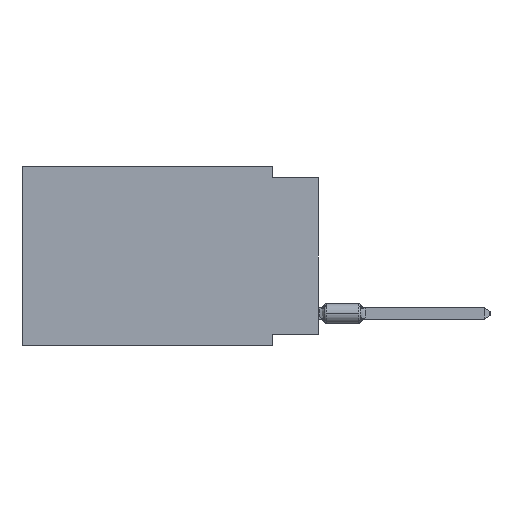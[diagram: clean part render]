
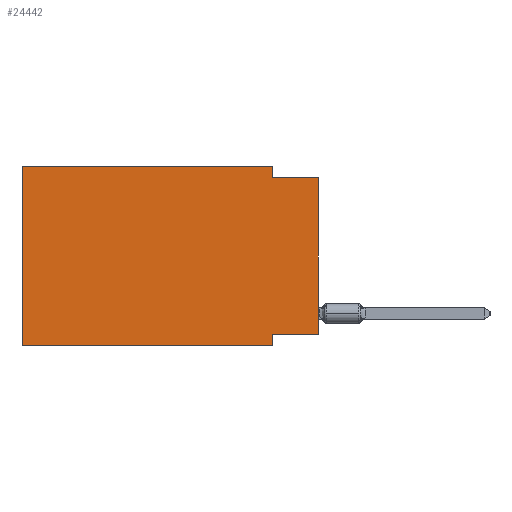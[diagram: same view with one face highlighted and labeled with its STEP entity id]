
A CAD part, left-side view. The second image highlights one B-rep face of the part: STEP entity #24442.
In plain terms, the highlighted planar face has unit normal (-1, 0, 0).
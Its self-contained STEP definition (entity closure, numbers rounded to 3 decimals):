
#1046 = AXIS2_PLACEMENT_3D ( 'NONE', #39281, #25412, #35504 ) ;
#1275 = CARTESIAN_POINT ( 'NONE',  ( 0., 16.383, 0. ) ) ;
#1671 = EDGE_CURVE ( 'NONE', #38551, #7655, #11116, .T. ) ;
#2085 = DIRECTION ( 'NONE',  ( 0., 0., 1. ) ) ;
#3081 = EDGE_CURVE ( 'NONE', #30205, #43479, #19618, .T. ) ;
#3796 = EDGE_CURVE ( 'NONE', #30205, #14501, #11627, .T. ) ;
#4505 = DIRECTION ( 'NONE',  ( 0., -1., 0. ) ) ;
#5519 = CARTESIAN_POINT ( 'NONE',  ( 0., 0., 0. ) ) ;
#6360 = CARTESIAN_POINT ( 'NONE',  ( 0., 2.54, -9.906 ) ) ;
#7655 = VERTEX_POINT ( 'NONE', #32848 ) ;
#8376 = FACE_OUTER_BOUND ( 'NONE', #14781, .T. ) ;
#8791 = CARTESIAN_POINT ( 'NONE',  ( 0., 2.54, 0. ) ) ;
#9458 = LINE ( 'NONE', #32788, #31918 ) ;
#10116 = CARTESIAN_POINT ( 'NONE',  ( 0., 2.54, -0.635 ) ) ;
#11116 = LINE ( 'NONE', #42030, #40801 ) ;
#11627 = LINE ( 'NONE', #22161, #36721 ) ;
#11852 = DIRECTION ( 'NONE',  ( 0., 1., 0. ) ) ;
#12559 = VECTOR ( 'NONE', #4505, 1000. ) ;
#12572 = VERTEX_POINT ( 'NONE', #10116 ) ;
#14501 = VERTEX_POINT ( 'NONE', #23857 ) ;
#14781 = EDGE_LOOP ( 'NONE', ( #31354, #17717, #36612, #36747, #33207, #42353, #42461, #24966 ) ) ;
#16635 = VECTOR ( 'NONE', #26085, 1000. ) ;
#17512 = LINE ( 'NONE', #41033, #32319 ) ;
#17717 = ORIENTED_EDGE ( 'NONE', *, *, #43012, .F. ) ;
#18783 = CARTESIAN_POINT ( 'NONE',  ( 0., 16.383, -9.906 ) ) ;
#19618 = LINE ( 'NONE', #5519, #23778 ) ;
#22090 = DIRECTION ( 'NONE',  ( 0., -1., 0. ) ) ;
#22161 = CARTESIAN_POINT ( 'NONE',  ( 0., 0., -9.271 ) ) ;
#23270 = EDGE_CURVE ( 'NONE', #14501, #30588, #39729, .T. ) ;
#23373 = DIRECTION ( 'NONE',  ( 0., 0., -1. ) ) ;
#23778 = VECTOR ( 'NONE', #25686, 1000. ) ;
#23857 = CARTESIAN_POINT ( 'NONE',  ( 0., 2.54, -9.271 ) ) ;
#23924 = CARTESIAN_POINT ( 'NONE',  ( 0., 0., -0.635 ) ) ;
#24442 = ADVANCED_FACE ( 'NONE', ( #8376 ), #35705, .F. ) ;
#24966 = ORIENTED_EDGE ( 'NONE', *, *, #3796, .F. ) ;
#25412 = DIRECTION ( 'NONE',  ( 1., 0., 0. ) ) ;
#25579 = VECTOR ( 'NONE', #23373, 1000. ) ;
#25686 = DIRECTION ( 'NONE',  ( 0., 0., 1. ) ) ;
#26085 = DIRECTION ( 'NONE',  ( 0., 0., -1. ) ) ;
#30205 = VERTEX_POINT ( 'NONE', #42338 ) ;
#30588 = VERTEX_POINT ( 'NONE', #41194 ) ;
#31191 = LINE ( 'NONE', #34539, #12559 ) ;
#31283 = EDGE_CURVE ( 'NONE', #34034, #30588, #31191, .T. ) ;
#31354 = ORIENTED_EDGE ( 'NONE', *, *, #3081, .T. ) ;
#31918 = VECTOR ( 'NONE', #2085, 1000. ) ;
#32319 = VECTOR ( 'NONE', #33668, 1000. ) ;
#32699 = EDGE_CURVE ( 'NONE', #7655, #12572, #36813, .T. ) ;
#32788 = CARTESIAN_POINT ( 'NONE',  ( 0., 16.383, 0. ) ) ;
#32848 = CARTESIAN_POINT ( 'NONE',  ( 0., 2.54, 0. ) ) ;
#33207 = ORIENTED_EDGE ( 'NONE', *, *, #42834, .F. ) ;
#33668 = DIRECTION ( 'NONE',  ( 0., -1., 0. ) ) ;
#34034 = VERTEX_POINT ( 'NONE', #18783 ) ;
#34539 = CARTESIAN_POINT ( 'NONE',  ( 0., 16.383, -9.906 ) ) ;
#35504 = DIRECTION ( 'NONE',  ( 0., 0., -1. ) ) ;
#35705 = PLANE ( 'NONE',  #1046 ) ;
#36612 = ORIENTED_EDGE ( 'NONE', *, *, #32699, .F. ) ;
#36721 = VECTOR ( 'NONE', #11852, 1000. ) ;
#36747 = ORIENTED_EDGE ( 'NONE', *, *, #1671, .F. ) ;
#36813 = LINE ( 'NONE', #8791, #25579 ) ;
#38551 = VERTEX_POINT ( 'NONE', #1275 ) ;
#39281 = CARTESIAN_POINT ( 'NONE',  ( 0., 16.383, 0. ) ) ;
#39729 = LINE ( 'NONE', #6360, #16635 ) ;
#40801 = VECTOR ( 'NONE', #22090, 1000. ) ;
#41033 = CARTESIAN_POINT ( 'NONE',  ( 0., 0., -0.635 ) ) ;
#41194 = CARTESIAN_POINT ( 'NONE',  ( 0., 2.54, -9.906 ) ) ;
#42030 = CARTESIAN_POINT ( 'NONE',  ( 0., 16.383, 0. ) ) ;
#42338 = CARTESIAN_POINT ( 'NONE',  ( 0., 0., -9.271 ) ) ;
#42353 = ORIENTED_EDGE ( 'NONE', *, *, #31283, .T. ) ;
#42461 = ORIENTED_EDGE ( 'NONE', *, *, #23270, .F. ) ;
#42834 = EDGE_CURVE ( 'NONE', #34034, #38551, #9458, .T. ) ;
#43012 = EDGE_CURVE ( 'NONE', #12572, #43479, #17512, .T. ) ;
#43479 = VERTEX_POINT ( 'NONE', #23924 ) ;
